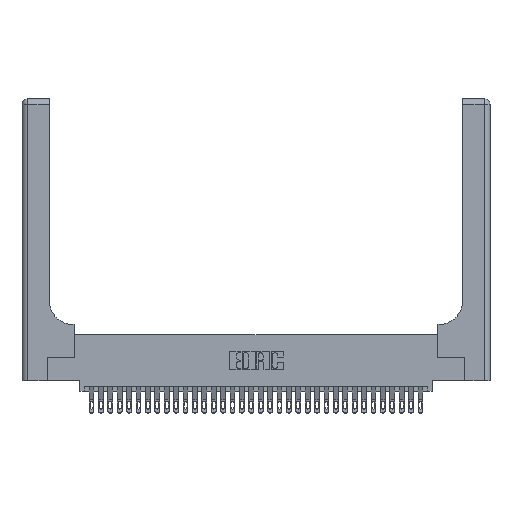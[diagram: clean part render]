
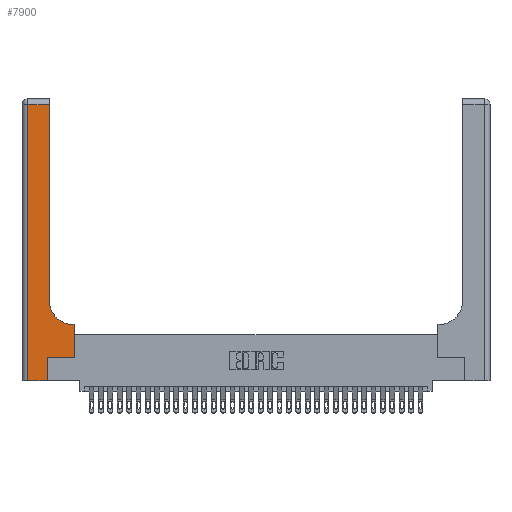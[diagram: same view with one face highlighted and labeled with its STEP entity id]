
A CAD part, top view. The second image highlights one B-rep face of the part: STEP entity #7900.
In plain terms, the highlighted planar face has unit normal (0, 0, 1).
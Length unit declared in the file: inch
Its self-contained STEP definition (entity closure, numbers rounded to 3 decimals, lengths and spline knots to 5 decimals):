
#47 = DIRECTION ( 'NONE',  ( -1., 0., 0. ) ) ;
#1446 = DIRECTION ( 'NONE',  ( -1., 0., 0. ) ) ;
#2008 = CARTESIAN_POINT ( 'NONE',  ( 0.2915, 0.85, 0.37 ) ) ;
#2168 = DIRECTION ( 'NONE',  ( -1., 0., 0. ) ) ;
#2481 = LINE ( 'NONE', #15024, #16274 ) ;
#2738 = ORIENTED_EDGE ( 'NONE', *, *, #7799, .T. ) ;
#3121 = CARTESIAN_POINT ( 'NONE',  ( 0.269, 0.25, 0.37 ) ) ;
#4626 = ORIENTED_EDGE ( 'NONE', *, *, #25545, .T. ) ;
#4739 = ORIENTED_EDGE ( 'NONE', *, *, #8403, .T. ) ;
#5097 = CARTESIAN_POINT ( 'NONE',  ( 0.5415, 0.6, 0.37 ) ) ;
#6236 = VECTOR ( 'NONE', #22187, 39.37008 ) ;
#6750 = CARTESIAN_POINT ( 'NONE',  ( 0.5415, 0.85, 0.37 ) ) ;
#6810 = VERTEX_POINT ( 'NONE', #19756 ) ;
#7189 = LINE ( 'NONE', #23887, #29008 ) ;
#7799 = EDGE_CURVE ( 'NONE', #11006, #14678, #25788, .T. ) ;
#7900 = ADVANCED_FACE ( 'NONE', ( #11489 ), #22908, .F. ) ;
#8403 = EDGE_CURVE ( 'NONE', #34069, #33103, #12721, .T. ) ;
#8746 = EDGE_CURVE ( 'NONE', #9529, #25896, #32787, .T. ) ;
#9529 = VERTEX_POINT ( 'NONE', #29017 ) ;
#9669 = CARTESIAN_POINT ( 'NONE',  ( 0.5585, 0.6, 0.37 ) ) ;
#10078 = ORIENTED_EDGE ( 'NONE', *, *, #31978, .T. ) ;
#10537 = DIRECTION ( 'NONE',  ( 0., -1., 0. ) ) ;
#11006 = VERTEX_POINT ( 'NONE', #2008 ) ;
#11489 = FACE_OUTER_BOUND ( 'NONE', #12517, .T. ) ;
#11717 = LINE ( 'NONE', #29728, #29378 ) ;
#12517 = EDGE_LOOP ( 'NONE', ( #2738, #19293, #4739, #10078, #26092, #23567, #18395, #32001, #4626 ) ) ;
#12721 = LINE ( 'NONE', #20995, #26543 ) ;
#14033 = DIRECTION ( 'NONE',  ( 0., 1., 0. ) ) ;
#14678 = VERTEX_POINT ( 'NONE', #20956 ) ;
#15024 = CARTESIAN_POINT ( 'NONE',  ( 0., 2.94, 0.37 ) ) ;
#15530 = VERTEX_POINT ( 'NONE', #5097 ) ;
#15768 = DIRECTION ( 'NONE',  ( 0., 1., 0. ) ) ;
#16256 = LINE ( 'NONE', #22523, #29727 ) ;
#16274 = VECTOR ( 'NONE', #1446, 39.37008 ) ;
#16893 = EDGE_CURVE ( 'NONE', #14678, #34069, #2481, .T. ) ;
#17731 = DIRECTION ( 'NONE',  ( 0., 0., -1. ) ) ;
#18395 = ORIENTED_EDGE ( 'NONE', *, *, #20907, .T. ) ;
#19130 = CARTESIAN_POINT ( 'NONE',  ( 0., 0., 0.37 ) ) ;
#19293 = ORIENTED_EDGE ( 'NONE', *, *, #16893, .T. ) ;
#19756 = CARTESIAN_POINT ( 'NONE',  ( 0.5585, 0.25, 0.37 ) ) ;
#20121 = CARTESIAN_POINT ( 'NONE',  ( 0.2915, 3., 0.37 ) ) ;
#20907 = EDGE_CURVE ( 'NONE', #6810, #28560, #16256, .T. ) ;
#20956 = CARTESIAN_POINT ( 'NONE',  ( 0.2915, 2.94, 0.37 ) ) ;
#20995 = CARTESIAN_POINT ( 'NONE',  ( 0.06, 3., 0.37 ) ) ;
#22187 = DIRECTION ( 'NONE',  ( 1., 0., 0. ) ) ;
#22296 = CIRCLE ( 'NONE', #24160, 0.25 ) ;
#22523 = CARTESIAN_POINT ( 'NONE',  ( 0.5585, 0.25, 0.37 ) ) ;
#22677 = AXIS2_PLACEMENT_3D ( 'NONE', #31913, #29025, #2168 ) ;
#22908 = PLANE ( 'NONE',  #22677 ) ;
#23567 = ORIENTED_EDGE ( 'NONE', *, *, #33619, .T. ) ;
#23887 = CARTESIAN_POINT ( 'NONE',  ( 0.269, 0.25, 0.37 ) ) ;
#24074 = VECTOR ( 'NONE', #15768, 39.37008 ) ;
#24160 = AXIS2_PLACEMENT_3D ( 'NONE', #6750, #17731, #25360 ) ;
#25104 = LINE ( 'NONE', #19130, #6236 ) ;
#25360 = DIRECTION ( 'NONE',  ( 1., 0., 0. ) ) ;
#25545 = EDGE_CURVE ( 'NONE', #15530, #11006, #22296, .T. ) ;
#25717 = VECTOR ( 'NONE', #14033, 39.37008 ) ;
#25788 = LINE ( 'NONE', #20121, #24074 ) ;
#25896 = VERTEX_POINT ( 'NONE', #3121 ) ;
#26092 = ORIENTED_EDGE ( 'NONE', *, *, #8746, .T. ) ;
#26543 = VECTOR ( 'NONE', #10537, 39.37008 ) ;
#26547 = CARTESIAN_POINT ( 'NONE',  ( 0.06, 2.94, 0.37 ) ) ;
#28560 = VERTEX_POINT ( 'NONE', #9669 ) ;
#29008 = VECTOR ( 'NONE', #29525, 39.37008 ) ;
#29017 = CARTESIAN_POINT ( 'NONE',  ( 0.269, 0., 0.37 ) ) ;
#29025 = DIRECTION ( 'NONE',  ( 0., 0., -1. ) ) ;
#29378 = VECTOR ( 'NONE', #47, 39.37008 ) ;
#29525 = DIRECTION ( 'NONE',  ( 1., 0., 0. ) ) ;
#29727 = VECTOR ( 'NONE', #30630, 39.37008 ) ;
#29728 = CARTESIAN_POINT ( 'NONE',  ( 0.2915, 0.6, 0.37 ) ) ;
#30245 = CARTESIAN_POINT ( 'NONE',  ( 0.06, 0., 0.37 ) ) ;
#30277 = CARTESIAN_POINT ( 'NONE',  ( 0.269, 0., 0.37 ) ) ;
#30630 = DIRECTION ( 'NONE',  ( 0., 1., 0. ) ) ;
#31462 = EDGE_CURVE ( 'NONE', #28560, #15530, #11717, .T. ) ;
#31913 = CARTESIAN_POINT ( 'NONE',  ( 0., 3., 0.37 ) ) ;
#31978 = EDGE_CURVE ( 'NONE', #33103, #9529, #25104, .T. ) ;
#32001 = ORIENTED_EDGE ( 'NONE', *, *, #31462, .T. ) ;
#32787 = LINE ( 'NONE', #30277, #25717 ) ;
#33103 = VERTEX_POINT ( 'NONE', #30245 ) ;
#33619 = EDGE_CURVE ( 'NONE', #25896, #6810, #7189, .T. ) ;
#34069 = VERTEX_POINT ( 'NONE', #26547 ) ;
